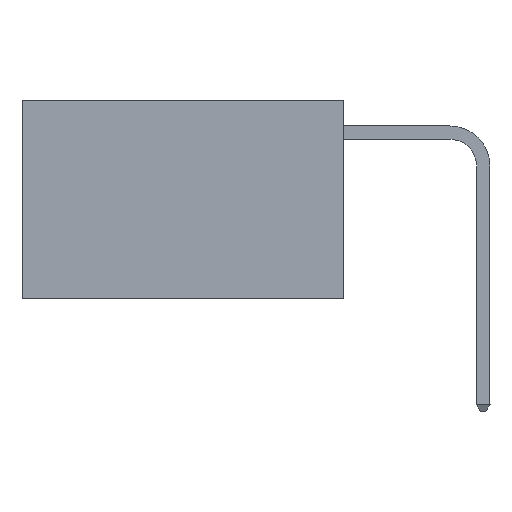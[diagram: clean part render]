
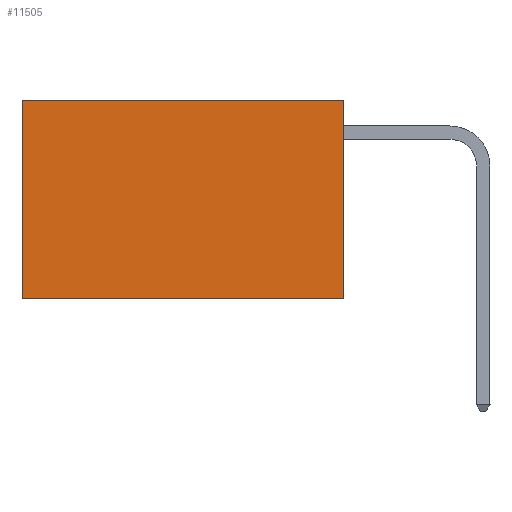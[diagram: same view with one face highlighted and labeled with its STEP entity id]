
A CAD part, left-side view. The second image highlights one B-rep face of the part: STEP entity #11505.
In plain terms, the highlighted planar face has unit normal (-1, 0, 0).
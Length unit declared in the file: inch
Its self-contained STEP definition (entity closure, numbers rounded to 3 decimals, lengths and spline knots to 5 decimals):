
#723 = EDGE_CURVE ( 'NONE', #22678, #5854, #1518, .T. ) ;
#1446 = EDGE_CURVE ( 'NONE', #11786, #22678, #23471, .T. ) ;
#1518 = LINE ( 'NONE', #13047, #3785 ) ;
#2304 = DIRECTION ( 'NONE',  ( 0., 1., 0. ) ) ;
#3116 = ORIENTED_EDGE ( 'NONE', *, *, #6579, .T. ) ;
#3575 = CARTESIAN_POINT ( 'NONE',  ( 0.2625, 0.6, -0.37 ) ) ;
#3785 = VECTOR ( 'NONE', #26983, 39.37008 ) ;
#5042 = FACE_OUTER_BOUND ( 'NONE', #22187, .T. ) ;
#5431 = AXIS2_PLACEMENT_3D ( 'NONE', #22725, #11302, #7158 ) ;
#5854 = VERTEX_POINT ( 'NONE', #3575 ) ;
#6102 = CARTESIAN_POINT ( 'NONE',  ( 0.2625, 0.6, 0. ) ) ;
#6579 = EDGE_CURVE ( 'NONE', #11786, #17849, #22981, .T. ) ;
#6705 = LINE ( 'NONE', #16638, #20457 ) ;
#7158 = DIRECTION ( 'NONE',  ( 0., 0., -1. ) ) ;
#10952 = CARTESIAN_POINT ( 'NONE',  ( 0.2625, 0., -0.37 ) ) ;
#11302 = DIRECTION ( 'NONE',  ( 1., 0., 0. ) ) ;
#11505 = ADVANCED_FACE ( 'NONE', ( #5042 ), #15828, .F. ) ;
#11786 = VERTEX_POINT ( 'NONE', #13066 ) ;
#13047 = CARTESIAN_POINT ( 'NONE',  ( 0.2625, 0., -0.37 ) ) ;
#13066 = CARTESIAN_POINT ( 'NONE',  ( 0.2625, 0., 0. ) ) ;
#13554 = ORIENTED_EDGE ( 'NONE', *, *, #723, .F. ) ;
#15047 = EDGE_CURVE ( 'NONE', #17849, #5854, #6705, .T. ) ;
#15369 = VECTOR ( 'NONE', #2304, 39.37008 ) ;
#15828 = PLANE ( 'NONE',  #5431 ) ;
#16638 = CARTESIAN_POINT ( 'NONE',  ( 0.2625, 0.6, 0. ) ) ;
#17849 = VERTEX_POINT ( 'NONE', #6102 ) ;
#20457 = VECTOR ( 'NONE', #25792, 39.37008 ) ;
#20496 = CARTESIAN_POINT ( 'NONE',  ( 0.2625, 0., 0. ) ) ;
#22187 = EDGE_LOOP ( 'NONE', ( #23283, #13554, #22894, #3116 ) ) ;
#22678 = VERTEX_POINT ( 'NONE', #10952 ) ;
#22725 = CARTESIAN_POINT ( 'NONE',  ( 0.2625, 0., 0. ) ) ;
#22894 = ORIENTED_EDGE ( 'NONE', *, *, #1446, .F. ) ;
#22981 = LINE ( 'NONE', #25662, #15369 ) ;
#23283 = ORIENTED_EDGE ( 'NONE', *, *, #15047, .T. ) ;
#23471 = LINE ( 'NONE', #20496, #27629 ) ;
#25662 = CARTESIAN_POINT ( 'NONE',  ( 0.2625, 0., 0. ) ) ;
#25792 = DIRECTION ( 'NONE',  ( 0., 0., -1. ) ) ;
#26983 = DIRECTION ( 'NONE',  ( 0., 1., 0. ) ) ;
#27629 = VECTOR ( 'NONE', #29644, 39.37008 ) ;
#29644 = DIRECTION ( 'NONE',  ( 0., 0., -1. ) ) ;
